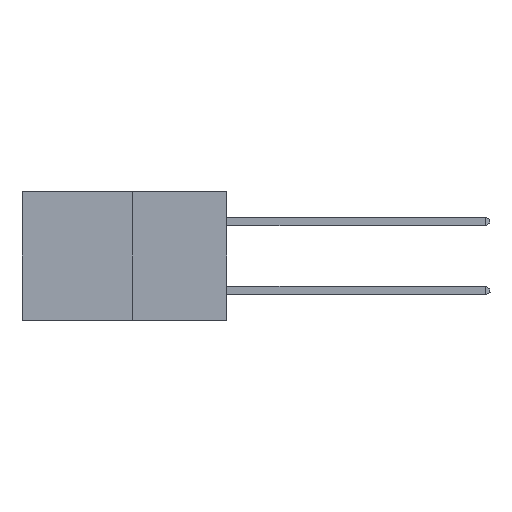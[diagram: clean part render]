
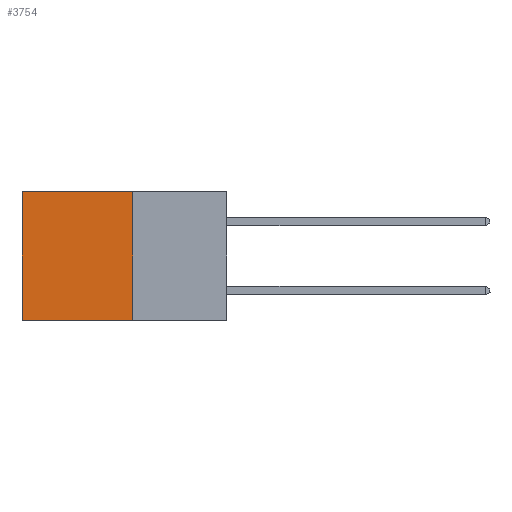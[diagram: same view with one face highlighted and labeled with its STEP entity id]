
A CAD part, left-side view. The second image highlights one B-rep face of the part: STEP entity #3754.
In plain terms, the highlighted planar face has unit normal (-1, 0, 0).
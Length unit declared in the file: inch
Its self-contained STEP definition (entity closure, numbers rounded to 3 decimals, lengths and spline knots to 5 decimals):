
#34 = VERTEX_POINT ( 'NONE', #1840 ) ;
#89 = DIRECTION ( 'NONE',  ( 0., 0., -1. ) ) ;
#147 = DIRECTION ( 'NONE',  ( 1., 0., 0. ) ) ;
#284 = ORIENTED_EDGE ( 'NONE', *, *, #6573, .T. ) ;
#1840 = CARTESIAN_POINT ( 'NONE',  ( 0.277, 0.59, 0. ) ) ;
#1878 = LINE ( 'NONE', #3262, #10146 ) ;
#2596 = EDGE_CURVE ( 'NONE', #3279, #5849, #1878, .T. ) ;
#3262 = CARTESIAN_POINT ( 'NONE',  ( 0.277, 0.27, -0.37 ) ) ;
#3279 = VERTEX_POINT ( 'NONE', #9460 ) ;
#3354 = ORIENTED_EDGE ( 'NONE', *, *, #2596, .F. ) ;
#3477 = DIRECTION ( 'NONE',  ( 0., 0., -1. ) ) ;
#3653 = VECTOR ( 'NONE', #6113, 39.37008 ) ;
#3754 = ADVANCED_FACE ( 'NONE', ( #7299 ), #8156, .F. ) ;
#3941 = LINE ( 'NONE', #5287, #3653 ) ;
#4258 = ORIENTED_EDGE ( 'NONE', *, *, #9609, .F. ) ;
#4380 = CARTESIAN_POINT ( 'NONE',  ( 0.277, 0.59, -0.37 ) ) ;
#4384 = LINE ( 'NONE', #4380, #8214 ) ;
#4962 = EDGE_LOOP ( 'NONE', ( #9396, #4258, #3354, #284 ) ) ;
#5287 = CARTESIAN_POINT ( 'NONE',  ( 0.277, 0.27, -0.37 ) ) ;
#5337 = DIRECTION ( 'NONE',  ( 0., 1., 0. ) ) ;
#5512 = CARTESIAN_POINT ( 'NONE',  ( 0.277, 0.27, 0. ) ) ;
#5633 = DIRECTION ( 'NONE',  ( 0., 0., -1. ) ) ;
#5849 = VERTEX_POINT ( 'NONE', #9261 ) ;
#6113 = DIRECTION ( 'NONE',  ( 0., 1., 0. ) ) ;
#6573 = EDGE_CURVE ( 'NONE', #3279, #34, #6901, .T. ) ;
#6901 = LINE ( 'NONE', #5512, #8139 ) ;
#7299 = FACE_OUTER_BOUND ( 'NONE', #4962, .T. ) ;
#7466 = AXIS2_PLACEMENT_3D ( 'NONE', #8176, #147, #89 ) ;
#7682 = VERTEX_POINT ( 'NONE', #7992 ) ;
#7992 = CARTESIAN_POINT ( 'NONE',  ( 0.277, 0.59, -0.37 ) ) ;
#8139 = VECTOR ( 'NONE', #5337, 39.37008 ) ;
#8156 = PLANE ( 'NONE',  #7466 ) ;
#8176 = CARTESIAN_POINT ( 'NONE',  ( 0.277, 0.27, -0.37 ) ) ;
#8214 = VECTOR ( 'NONE', #3477, 39.37008 ) ;
#8804 = EDGE_CURVE ( 'NONE', #34, #7682, #4384, .T. ) ;
#9261 = CARTESIAN_POINT ( 'NONE',  ( 0.277, 0.27, -0.37 ) ) ;
#9396 = ORIENTED_EDGE ( 'NONE', *, *, #8804, .T. ) ;
#9460 = CARTESIAN_POINT ( 'NONE',  ( 0.277, 0.27, 0. ) ) ;
#9609 = EDGE_CURVE ( 'NONE', #5849, #7682, #3941, .T. ) ;
#10146 = VECTOR ( 'NONE', #5633, 39.37008 ) ;
